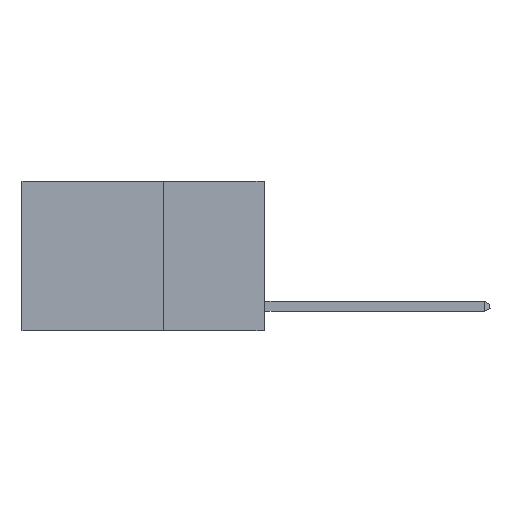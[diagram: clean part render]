
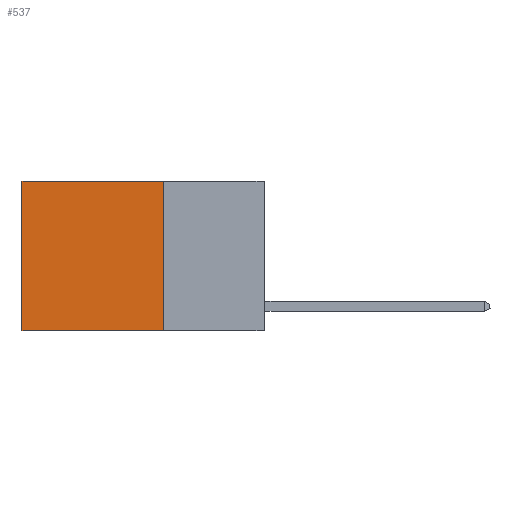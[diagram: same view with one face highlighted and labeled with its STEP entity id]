
A CAD part, left-side view. The second image highlights one B-rep face of the part: STEP entity #537.
In plain terms, the highlighted planar face has unit normal (-1, 0, 0).
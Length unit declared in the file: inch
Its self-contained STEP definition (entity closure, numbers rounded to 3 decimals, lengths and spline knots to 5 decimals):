
#461 = CARTESIAN_POINT ( 'NONE',  ( 0.2625, 0.25, 0. ) ) ;
#537 = ADVANCED_FACE ( 'NONE', ( #12303 ), #1028, .F. ) ;
#1028 = PLANE ( 'NONE',  #8089 ) ;
#1683 = LINE ( 'NONE', #12923, #2846 ) ;
#2846 = VECTOR ( 'NONE', #10906, 39.37008 ) ;
#2855 = CARTESIAN_POINT ( 'NONE',  ( 0.2625, 0.6, -0.37 ) ) ;
#3028 = DIRECTION ( 'NONE',  ( 1., 0., 0. ) ) ;
#3213 = DIRECTION ( 'NONE',  ( 0., 0., -1. ) ) ;
#3291 = EDGE_CURVE ( 'NONE', #12583, #7382, #1683, .T. ) ;
#4085 = LINE ( 'NONE', #5140, #10713 ) ;
#4928 = CARTESIAN_POINT ( 'NONE',  ( 0.2625, 0.25, 0. ) ) ;
#5140 = CARTESIAN_POINT ( 'NONE',  ( 0.2625, 0.6, 0. ) ) ;
#5229 = CARTESIAN_POINT ( 'NONE',  ( 0.2625, 0.25, -0.37 ) ) ;
#5346 = ORIENTED_EDGE ( 'NONE', *, *, #3291, .T. ) ;
#5567 = VERTEX_POINT ( 'NONE', #2855 ) ;
#5800 = DIRECTION ( 'NONE',  ( 0., 0., -1. ) ) ;
#6489 = DIRECTION ( 'NONE',  ( 0., 1., 0. ) ) ;
#6895 = EDGE_CURVE ( 'NONE', #7382, #5567, #4085, .T. ) ;
#7382 = VERTEX_POINT ( 'NONE', #11788 ) ;
#7506 = DIRECTION ( 'NONE',  ( 0., 0., -1. ) ) ;
#8089 = AXIS2_PLACEMENT_3D ( 'NONE', #4928, #3028, #5800 ) ;
#8540 = ORIENTED_EDGE ( 'NONE', *, *, #12544, .F. ) ;
#8804 = LINE ( 'NONE', #11690, #10888 ) ;
#9318 = CARTESIAN_POINT ( 'NONE',  ( 0.2625, 0.25, 0. ) ) ;
#9622 = ORIENTED_EDGE ( 'NONE', *, *, #11068, .F. ) ;
#10298 = EDGE_LOOP ( 'NONE', ( #10939, #8540, #9622, #5346 ) ) ;
#10713 = VECTOR ( 'NONE', #7506, 39.37008 ) ;
#10720 = VECTOR ( 'NONE', #3213, 39.37008 ) ;
#10888 = VECTOR ( 'NONE', #6489, 39.37008 ) ;
#10906 = DIRECTION ( 'NONE',  ( 0., 1., 0. ) ) ;
#10939 = ORIENTED_EDGE ( 'NONE', *, *, #6895, .T. ) ;
#11068 = EDGE_CURVE ( 'NONE', #12583, #13167, #11529, .T. ) ;
#11529 = LINE ( 'NONE', #461, #10720 ) ;
#11690 = CARTESIAN_POINT ( 'NONE',  ( 0.2625, 0.25, -0.37 ) ) ;
#11788 = CARTESIAN_POINT ( 'NONE',  ( 0.2625, 0.6, 0. ) ) ;
#12303 = FACE_OUTER_BOUND ( 'NONE', #10298, .T. ) ;
#12544 = EDGE_CURVE ( 'NONE', #13167, #5567, #8804, .T. ) ;
#12583 = VERTEX_POINT ( 'NONE', #9318 ) ;
#12923 = CARTESIAN_POINT ( 'NONE',  ( 0.2625, 0.25, 0. ) ) ;
#13167 = VERTEX_POINT ( 'NONE', #5229 ) ;
